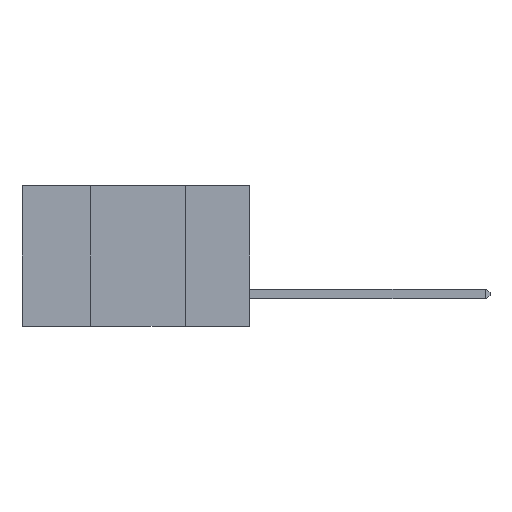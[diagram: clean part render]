
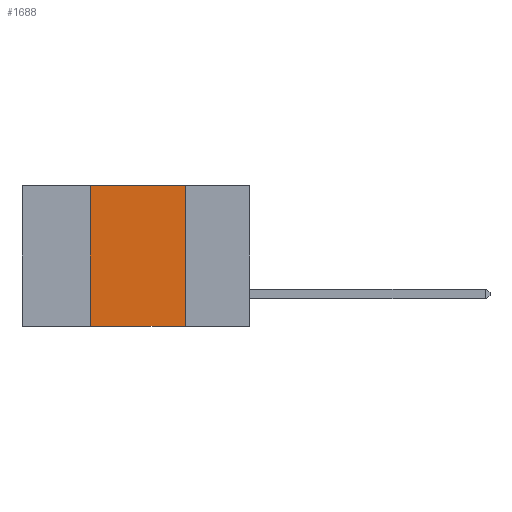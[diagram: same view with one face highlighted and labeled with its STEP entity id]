
A CAD part, left-side view. The second image highlights one B-rep face of the part: STEP entity #1688.
In plain terms, the highlighted planar face has unit normal (-1, 0, 0).
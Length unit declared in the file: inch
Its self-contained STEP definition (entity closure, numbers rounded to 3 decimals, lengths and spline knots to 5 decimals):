
#93 = CARTESIAN_POINT ( 'NONE',  ( 0., 0.42, 0. ) ) ;
#1407 = VECTOR ( 'NONE', #3329, 39.37008 ) ;
#1600 = EDGE_CURVE ( 'NONE', #9437, #10312, #4617, .T. ) ;
#1688 = ADVANCED_FACE ( 'NONE', ( #6141 ), #11594, .F. ) ;
#1941 = LINE ( 'NONE', #10323, #7357 ) ;
#1999 = EDGE_CURVE ( 'NONE', #10312, #8219, #5957, .T. ) ;
#2687 = DIRECTION ( 'NONE',  ( 0., 0., -1. ) ) ;
#3095 = VERTEX_POINT ( 'NONE', #10808 ) ;
#3329 = DIRECTION ( 'NONE',  ( 0., 0., 1. ) ) ;
#4617 = LINE ( 'NONE', #5290, #9548 ) ;
#5111 = DIRECTION ( 'NONE',  ( 0., -1., 0. ) ) ;
#5290 = CARTESIAN_POINT ( 'NONE',  ( 0., 0.6, 0. ) ) ;
#5957 = LINE ( 'NONE', #9035, #10809 ) ;
#6141 = FACE_OUTER_BOUND ( 'NONE', #7813, .T. ) ;
#6531 = DIRECTION ( 'NONE',  ( 1., 0., 0. ) ) ;
#7357 = VECTOR ( 'NONE', #5111, 39.37008 ) ;
#7813 = EDGE_LOOP ( 'NONE', ( #8555, #8635, #8661, #8737 ) ) ;
#8219 = VERTEX_POINT ( 'NONE', #10082 ) ;
#8555 = ORIENTED_EDGE ( 'NONE', *, *, #1999, .F. ) ;
#8635 = ORIENTED_EDGE ( 'NONE', *, *, #1600, .F. ) ;
#8661 = ORIENTED_EDGE ( 'NONE', *, *, #11366, .F. ) ;
#8737 = ORIENTED_EDGE ( 'NONE', *, *, #11121, .T. ) ;
#8829 = AXIS2_PLACEMENT_3D ( 'NONE', #10622, #6531, #13536 ) ;
#9035 = CARTESIAN_POINT ( 'NONE',  ( 0., 0.17, 0. ) ) ;
#9078 = CARTESIAN_POINT ( 'NONE',  ( 0., 0.17, 0. ) ) ;
#9437 = VERTEX_POINT ( 'NONE', #9835 ) ;
#9548 = VECTOR ( 'NONE', #13447, 39.37008 ) ;
#9835 = CARTESIAN_POINT ( 'NONE',  ( 0., 0.42, 0. ) ) ;
#9915 = LINE ( 'NONE', #93, #1407 ) ;
#10082 = CARTESIAN_POINT ( 'NONE',  ( 0., 0.17, -0.37 ) ) ;
#10312 = VERTEX_POINT ( 'NONE', #9078 ) ;
#10323 = CARTESIAN_POINT ( 'NONE',  ( 0., 0.6, -0.37 ) ) ;
#10622 = CARTESIAN_POINT ( 'NONE',  ( 0., 0.6, 0. ) ) ;
#10808 = CARTESIAN_POINT ( 'NONE',  ( 0., 0.42, -0.37 ) ) ;
#10809 = VECTOR ( 'NONE', #2687, 39.37008 ) ;
#11121 = EDGE_CURVE ( 'NONE', #3095, #8219, #1941, .T. ) ;
#11366 = EDGE_CURVE ( 'NONE', #3095, #9437, #9915, .T. ) ;
#11594 = PLANE ( 'NONE',  #8829 ) ;
#13447 = DIRECTION ( 'NONE',  ( 0., -1., 0. ) ) ;
#13536 = DIRECTION ( 'NONE',  ( 0., 0., -1. ) ) ;
